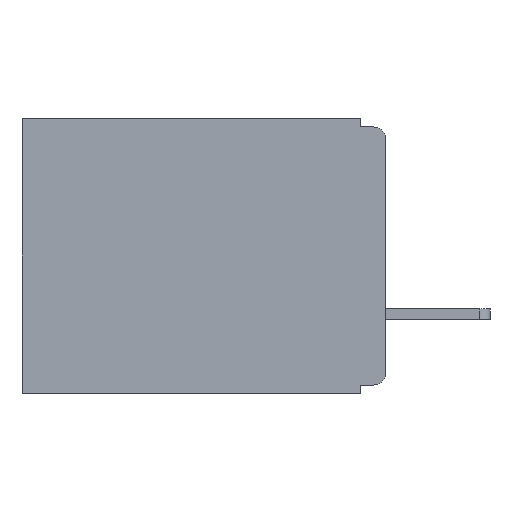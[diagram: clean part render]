
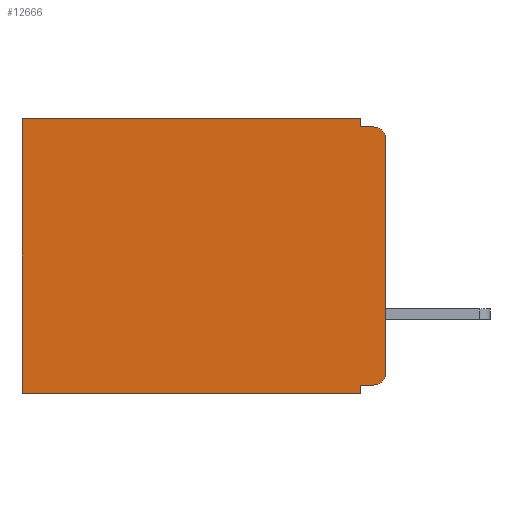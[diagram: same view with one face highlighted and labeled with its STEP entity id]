
A CAD part, left-side view. The second image highlights one B-rep face of the part: STEP entity #12666.
In plain terms, the highlighted planar face has unit normal (-1, 0, 0).
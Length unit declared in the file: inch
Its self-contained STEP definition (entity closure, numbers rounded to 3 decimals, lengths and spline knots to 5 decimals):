
#111 = VECTOR ( 'NONE', #9744, 39.37008 ) ;
#515 = VECTOR ( 'NONE', #8306, 39.37008 ) ;
#834 = CARTESIAN_POINT ( 'NONE',  ( 0.3, 0.437, -0.33 ) ) ;
#1118 = CARTESIAN_POINT ( 'NONE',  ( 0.3, 0.031, 0. ) ) ;
#1233 = CIRCLE ( 'NONE', #3289, 0.015 ) ;
#1372 = DIRECTION ( 'NONE',  ( -1., 0., 0. ) ) ;
#1430 = LINE ( 'NONE', #11179, #4269 ) ;
#1510 = CARTESIAN_POINT ( 'NONE',  ( 0.3, 0., -0.33 ) ) ;
#1546 = EDGE_CURVE ( 'NONE', #9440, #7468, #12158, .T. ) ;
#1626 = CIRCLE ( 'NONE', #3348, 0.015 ) ;
#1946 = CARTESIAN_POINT ( 'NONE',  ( 0.3, 0., 0. ) ) ;
#1982 = ORIENTED_EDGE ( 'NONE', *, *, #9505, .F. ) ;
#2040 = DIRECTION ( 'NONE',  ( 0., 0., -1. ) ) ;
#2048 = ORIENTED_EDGE ( 'NONE', *, *, #4423, .T. ) ;
#2055 = FACE_OUTER_BOUND ( 'NONE', #2833, .T. ) ;
#2161 = CARTESIAN_POINT ( 'NONE',  ( 0.3, 0.031, 0. ) ) ;
#2333 = ORIENTED_EDGE ( 'NONE', *, *, #10187, .T. ) ;
#2452 = VERTEX_POINT ( 'NONE', #12903 ) ;
#2467 = DIRECTION ( 'NONE',  ( 0., 1., 0. ) ) ;
#2833 = EDGE_LOOP ( 'NONE', ( #1982, #8888, #9539, #5316, #3986, #2048, #8115, #4125, #6594, #2333 ) ) ;
#3289 = AXIS2_PLACEMENT_3D ( 'NONE', #8191, #1372, #9280 ) ;
#3339 = LINE ( 'NONE', #5381, #111 ) ;
#3348 = AXIS2_PLACEMENT_3D ( 'NONE', #12088, #5944, #12941 ) ;
#3610 = VERTEX_POINT ( 'NONE', #11400 ) ;
#3707 = PLANE ( 'NONE',  #12106 ) ;
#3986 = ORIENTED_EDGE ( 'NONE', *, *, #1546, .T. ) ;
#4125 = ORIENTED_EDGE ( 'NONE', *, *, #13261, .F. ) ;
#4269 = VECTOR ( 'NONE', #2040, 39.37008 ) ;
#4423 = EDGE_CURVE ( 'NONE', #7468, #9902, #1430, .T. ) ;
#4624 = CARTESIAN_POINT ( 'NONE',  ( 0.3, 0.437, 0. ) ) ;
#5308 = VECTOR ( 'NONE', #7004, 39.37008 ) ;
#5316 = ORIENTED_EDGE ( 'NONE', *, *, #13242, .F. ) ;
#5381 = CARTESIAN_POINT ( 'NONE',  ( 0.3, 0., -0.01 ) ) ;
#5680 = DIRECTION ( 'NONE',  ( 0., 0., -1. ) ) ;
#5762 = DIRECTION ( 'NONE',  ( 0., 1., 0. ) ) ;
#5826 = VECTOR ( 'NONE', #10856, 39.37008 ) ;
#5927 = DIRECTION ( 'NONE',  ( 1., 0., 0. ) ) ;
#5944 = DIRECTION ( 'NONE',  ( -1., 0., 0. ) ) ;
#6136 = LINE ( 'NONE', #2161, #5826 ) ;
#6449 = CARTESIAN_POINT ( 'NONE',  ( 0.3, 0.031, -0.01 ) ) ;
#6594 = ORIENTED_EDGE ( 'NONE', *, *, #10059, .F. ) ;
#6722 = VECTOR ( 'NONE', #2467, 39.37008 ) ;
#7004 = DIRECTION ( 'NONE',  ( 0., 0., -1. ) ) ;
#7014 = VERTEX_POINT ( 'NONE', #7093 ) ;
#7093 = CARTESIAN_POINT ( 'NONE',  ( 0.3, 0.031, -0.32 ) ) ;
#7468 = VERTEX_POINT ( 'NONE', #4624 ) ;
#8115 = ORIENTED_EDGE ( 'NONE', *, *, #12835, .F. ) ;
#8191 = CARTESIAN_POINT ( 'NONE',  ( 0.3, 0.015, -0.305 ) ) ;
#8306 = DIRECTION ( 'NONE',  ( 0., 1., 0. ) ) ;
#8701 = VECTOR ( 'NONE', #5762, 39.37008 ) ;
#8888 = ORIENTED_EDGE ( 'NONE', *, *, #10150, .T. ) ;
#8981 = VERTEX_POINT ( 'NONE', #11188 ) ;
#9112 = VERTEX_POINT ( 'NONE', #12313 ) ;
#9188 = VERTEX_POINT ( 'NONE', #6449 ) ;
#9280 = DIRECTION ( 'NONE',  ( 0., 0., -1. ) ) ;
#9440 = VERTEX_POINT ( 'NONE', #1118 ) ;
#9505 = EDGE_CURVE ( 'NONE', #3610, #2452, #12758, .T. ) ;
#9539 = ORIENTED_EDGE ( 'NONE', *, *, #9817, .F. ) ;
#9569 = LINE ( 'NONE', #1510, #515 ) ;
#9744 = DIRECTION ( 'NONE',  ( 0., -1., 0. ) ) ;
#9817 = EDGE_CURVE ( 'NONE', #9188, #9112, #3339, .T. ) ;
#9902 = VERTEX_POINT ( 'NONE', #834 ) ;
#10059 = EDGE_CURVE ( 'NONE', #11869, #7014, #11331, .T. ) ;
#10150 = EDGE_CURVE ( 'NONE', #3610, #9112, #1626, .T. ) ;
#10187 = EDGE_CURVE ( 'NONE', #11869, #2452, #1233, .T. ) ;
#10856 = DIRECTION ( 'NONE',  ( 0., 0., -1. ) ) ;
#10976 = CARTESIAN_POINT ( 'NONE',  ( 0.3, 0., -0.32 ) ) ;
#11007 = CARTESIAN_POINT ( 'NONE',  ( 0.3, 0., -0.33 ) ) ;
#11057 = LINE ( 'NONE', #11848, #13396 ) ;
#11179 = CARTESIAN_POINT ( 'NONE',  ( 0.3, 0.437, -0.33 ) ) ;
#11188 = CARTESIAN_POINT ( 'NONE',  ( 0.3, 0.031, -0.33 ) ) ;
#11331 = LINE ( 'NONE', #10976, #8701 ) ;
#11400 = CARTESIAN_POINT ( 'NONE',  ( 0.3, 0., -0.025 ) ) ;
#11848 = CARTESIAN_POINT ( 'NONE',  ( 0.3, 0.031, -0.33 ) ) ;
#11869 = VERTEX_POINT ( 'NONE', #12543 ) ;
#12088 = CARTESIAN_POINT ( 'NONE',  ( 0.3, 0.015, -0.025 ) ) ;
#12106 = AXIS2_PLACEMENT_3D ( 'NONE', #11007, #5927, #12929 ) ;
#12158 = LINE ( 'NONE', #1946, #6722 ) ;
#12313 = CARTESIAN_POINT ( 'NONE',  ( 0.3, 0.015, -0.01 ) ) ;
#12543 = CARTESIAN_POINT ( 'NONE',  ( 0.3, 0.015, -0.32 ) ) ;
#12666 = ADVANCED_FACE ( 'NONE', ( #2055 ), #3707, .F. ) ;
#12758 = LINE ( 'NONE', #12953, #5308 ) ;
#12835 = EDGE_CURVE ( 'NONE', #8981, #9902, #9569, .T. ) ;
#12903 = CARTESIAN_POINT ( 'NONE',  ( 0.3, 0., -0.305 ) ) ;
#12929 = DIRECTION ( 'NONE',  ( 0., 0., -1. ) ) ;
#12941 = DIRECTION ( 'NONE',  ( 0., 0., -1. ) ) ;
#12953 = CARTESIAN_POINT ( 'NONE',  ( 0.3, 0., -0.33 ) ) ;
#13242 = EDGE_CURVE ( 'NONE', #9440, #9188, #6136, .T. ) ;
#13261 = EDGE_CURVE ( 'NONE', #7014, #8981, #11057, .T. ) ;
#13396 = VECTOR ( 'NONE', #5680, 39.37008 ) ;
